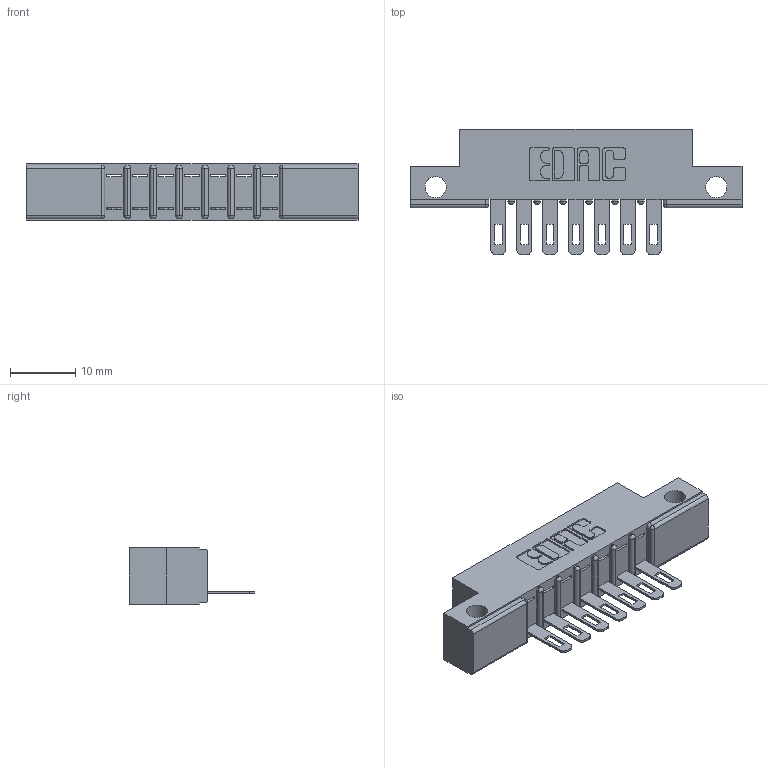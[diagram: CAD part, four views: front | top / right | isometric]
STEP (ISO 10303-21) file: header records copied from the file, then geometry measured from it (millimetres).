
FILE_DESCRIPTION (( 'STEP AP203' ), '1' );
FILE_NAME ('307-007-405-112.STEP', '2020-09-25T01:14:05', ( '' ), ( '' ), 'SwSTEP 2.0', 'SolidWorks 2020', '' );
FILE_SCHEMA (( 'CONFIG_CONTROL_DESIGN' ));
Length unit declared in the file: inch
Products named in the file (3): 307-290-001_505; 307 Part_.128 Dia Side Mounting Holes; 307-007-405-112
Assembly tree (8 placements, depth 2):
  307-007-405-112
    307 Part_.128 Dia Side Mounting Holes
    307-290-001_505  x7
Bounding box: 50.75 x 19.18 x 8.71 mm (x, y, z)
Volume: 3175.1 mm3; surface area: 4265.6 mm2
Topology: 8 solids, 8 shells, 518 faces, 1457 edges, 938 vertices
Faces by surface type: plane 322, cylinder 180, sphere 16
Entity records: 10292 total; most frequent: CARTESIAN_POINT 1720, ORIENTED_EDGE 1706, DIRECTION 1695, EDGE_CURVE 853, LINE 637, VECTOR 637, VERTEX_POINT 554, AXIS2_PLACEMENT_3D 529
